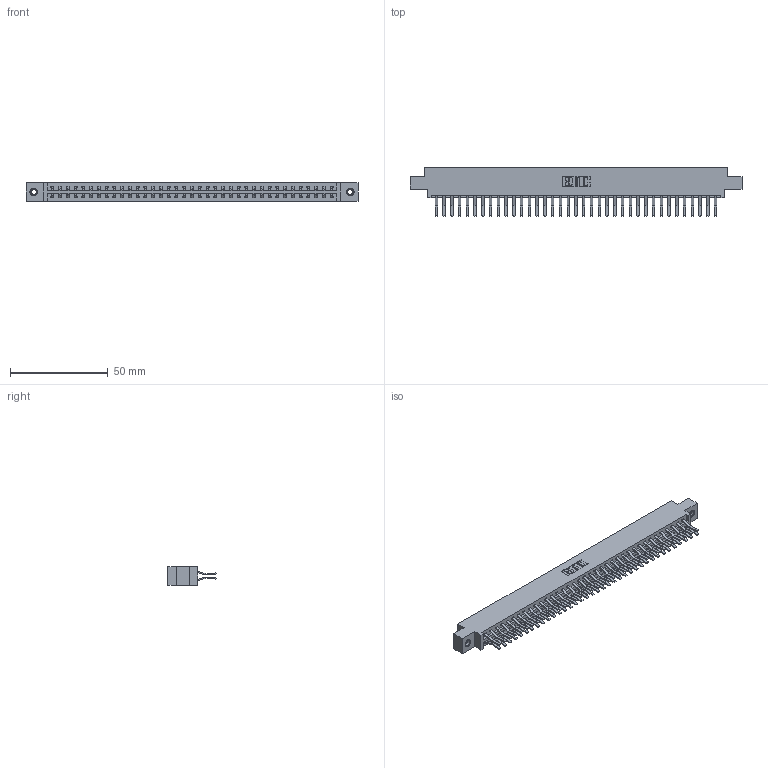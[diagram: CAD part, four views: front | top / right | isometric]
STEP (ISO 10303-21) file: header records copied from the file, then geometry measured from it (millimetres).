
FILE_DESCRIPTION (( 'STEP AP203' ), '1' );
FILE_NAME ('387-074-560-807.STEP', '2018-09-22T20:51:09', ( '' ), ( '' ), 'SwSTEP 2.0', 'SolidWorks 2016', '' );
FILE_SCHEMA (( 'CONFIG_CONTROL_DESIGN' ));
Length unit declared in the file: inch
Products named in the file (4): 337 Part_0.170 Offset - 0.156 Dia-TI; 345-292-001_560 Tail; 345-250-001_345-250-005-103; 387-074-560-807
Assembly tree (77 placements, depth 2):
  387-074-560-807
    337 Part_0.170 Offset - 0.156 Dia-TI
    345-292-001_560 Tail  x74
    345-250-001_345-250-005-103  x2
Bounding box: 169.62 x 24.78 x 9.4 mm (x, y, z)
Volume: 18163.5 mm3; surface area: 22032.9 mm2
Topology: 77 solids, 77 shells, 4322 faces, 12817 edges, 8438 vertices
Faces by surface type: plane 2918, cylinder 1388, cone 12, torus 4
Entity records: 30740 total; most frequent: CARTESIAN_POINT 5165, ORIENTED_EDGE 5094, DIRECTION 4437, EDGE_CURVE 2547, LINE 2395, VECTOR 2395, VERTEX_POINT 1692, AXIS2_PLACEMENT_3D 1021
